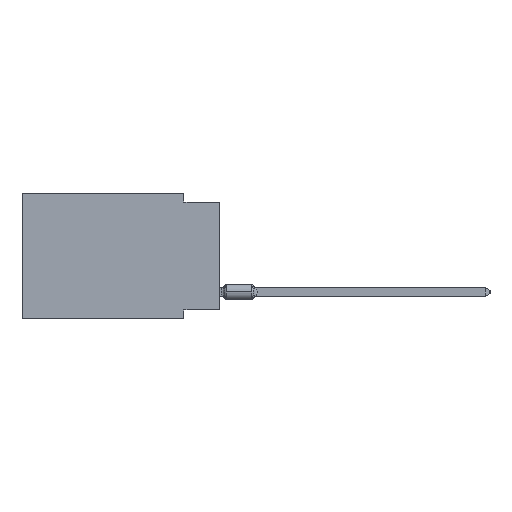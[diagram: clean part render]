
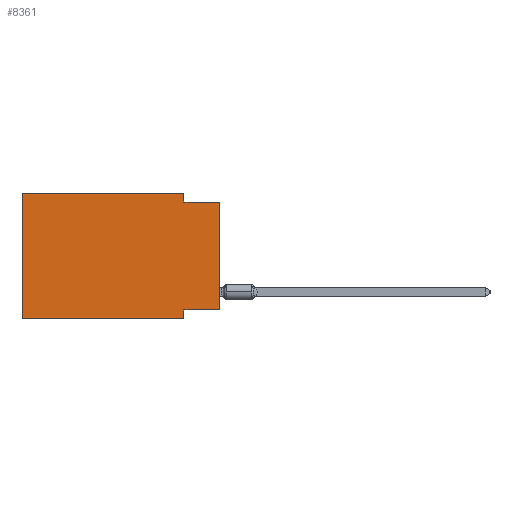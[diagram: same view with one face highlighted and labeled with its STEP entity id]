
A CAD part, left-side view. The second image highlights one B-rep face of the part: STEP entity #8361.
In plain terms, the highlighted planar face has unit normal (-1, 0, 0).
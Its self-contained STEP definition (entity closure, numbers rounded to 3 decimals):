
#645 = CARTESIAN_POINT ( 'NONE',  ( 0., 13.97, 0. ) ) ;
#853 = VERTEX_POINT ( 'NONE', #16847 ) ;
#8361 = ADVANCED_FACE ( 'NONE', ( #31615 ), #17648, .F. ) ;
#8714 = ORIENTED_EDGE ( 'NONE', *, *, #82675, .F. ) ;
#8896 = LINE ( 'NONE', #38214, #15114 ) ;
#10444 = DIRECTION ( 'NONE',  ( 0., -1., 0. ) ) ;
#12498 = VERTEX_POINT ( 'NONE', #42478 ) ;
#15114 = VECTOR ( 'NONE', #44915, 1000. ) ;
#16812 = CARTESIAN_POINT ( 'NONE',  ( 0., 2.54, -0.635 ) ) ;
#16847 = CARTESIAN_POINT ( 'NONE',  ( 0., 2.54, -8.89 ) ) ;
#17648 = PLANE ( 'NONE',  #80894 ) ;
#18167 = LINE ( 'NONE', #92196, #26492 ) ;
#18285 = CARTESIAN_POINT ( 'NONE',  ( 0., 2.54, -8.89 ) ) ;
#18522 = VECTOR ( 'NONE', #79520, 1000. ) ;
#21194 = DIRECTION ( 'NONE',  ( 0., 0., 1. ) ) ;
#21712 = ORIENTED_EDGE ( 'NONE', *, *, #71536, .F. ) ;
#26492 = VECTOR ( 'NONE', #47941, 1000. ) ;
#26695 = VECTOR ( 'NONE', #54966, 1000. ) ;
#28000 = CARTESIAN_POINT ( 'NONE',  ( 0., 0., -0.635 ) ) ;
#29479 = CARTESIAN_POINT ( 'NONE',  ( 0., 13.97, -8.89 ) ) ;
#30672 = CARTESIAN_POINT ( 'NONE',  ( 0., 13.97, -8.89 ) ) ;
#31040 = EDGE_CURVE ( 'NONE', #41817, #72069, #8896, .T. ) ;
#31063 = VERTEX_POINT ( 'NONE', #31460 ) ;
#31460 = CARTESIAN_POINT ( 'NONE',  ( 0., 2.54, 0. ) ) ;
#31615 = FACE_OUTER_BOUND ( 'NONE', #59789, .T. ) ;
#32337 = VECTOR ( 'NONE', #63117, 1000. ) ;
#34935 = CARTESIAN_POINT ( 'NONE',  ( 0., 13.97, 0. ) ) ;
#35223 = LINE ( 'NONE', #28000, #32337 ) ;
#38214 = CARTESIAN_POINT ( 'NONE',  ( 0., 13.97, 0. ) ) ;
#41817 = VERTEX_POINT ( 'NONE', #30672 ) ;
#42478 = CARTESIAN_POINT ( 'NONE',  ( 0., 2.54, -8.255 ) ) ;
#44915 = DIRECTION ( 'NONE',  ( 0., 0., 1. ) ) ;
#45713 = ORIENTED_EDGE ( 'NONE', *, *, #48249, .F. ) ;
#47765 = ORIENTED_EDGE ( 'NONE', *, *, #78366, .T. ) ;
#47941 = DIRECTION ( 'NONE',  ( 0., 1., 0. ) ) ;
#48249 = EDGE_CURVE ( 'NONE', #72069, #31063, #83504, .T. ) ;
#48394 = DIRECTION ( 'NONE',  ( 1., 0., 0. ) ) ;
#48626 = EDGE_CURVE ( 'NONE', #92317, #70538, #35223, .T. ) ;
#49755 = ORIENTED_EDGE ( 'NONE', *, *, #31040, .F. ) ;
#49796 = DIRECTION ( 'NONE',  ( 0., 0., -1. ) ) ;
#51533 = VERTEX_POINT ( 'NONE', #65725 ) ;
#52655 = VECTOR ( 'NONE', #75048, 1000. ) ;
#53529 = CARTESIAN_POINT ( 'NONE',  ( 0., 2.54, 0. ) ) ;
#53701 = CARTESIAN_POINT ( 'NONE',  ( 0., 13.97, 0. ) ) ;
#54966 = DIRECTION ( 'NONE',  ( 0., 0., -1. ) ) ;
#58596 = EDGE_CURVE ( 'NONE', #51533, #70538, #73563, .T. ) ;
#59789 = EDGE_LOOP ( 'NONE', ( #88439, #79707, #88510, #45713, #49755, #47765, #8714, #21712 ) ) ;
#61432 = VECTOR ( 'NONE', #10444, 1000. ) ;
#61665 = CARTESIAN_POINT ( 'NONE',  ( 0., 0., -0.635 ) ) ;
#63117 = DIRECTION ( 'NONE',  ( 0., -1., 0. ) ) ;
#64993 = VECTOR ( 'NONE', #21194, 1000. ) ;
#65725 = CARTESIAN_POINT ( 'NONE',  ( 0., 0., -8.255 ) ) ;
#68782 = LINE ( 'NONE', #18285, #52655 ) ;
#70538 = VERTEX_POINT ( 'NONE', #61665 ) ;
#71536 = EDGE_CURVE ( 'NONE', #51533, #12498, #18167, .T. ) ;
#72069 = VERTEX_POINT ( 'NONE', #645 ) ;
#73563 = LINE ( 'NONE', #87060, #64993 ) ;
#74659 = EDGE_CURVE ( 'NONE', #31063, #92317, #75170, .T. ) ;
#75048 = DIRECTION ( 'NONE',  ( 0., 0., -1. ) ) ;
#75170 = LINE ( 'NONE', #53529, #26695 ) ;
#78366 = EDGE_CURVE ( 'NONE', #41817, #853, #86726, .T. ) ;
#79520 = DIRECTION ( 'NONE',  ( 0., -1., 0. ) ) ;
#79707 = ORIENTED_EDGE ( 'NONE', *, *, #48626, .F. ) ;
#80894 = AXIS2_PLACEMENT_3D ( 'NONE', #34935, #48394, #49796 ) ;
#82675 = EDGE_CURVE ( 'NONE', #12498, #853, #68782, .T. ) ;
#83504 = LINE ( 'NONE', #53701, #61432 ) ;
#86726 = LINE ( 'NONE', #29479, #18522 ) ;
#87060 = CARTESIAN_POINT ( 'NONE',  ( 0., 0., 0. ) ) ;
#88439 = ORIENTED_EDGE ( 'NONE', *, *, #58596, .T. ) ;
#88510 = ORIENTED_EDGE ( 'NONE', *, *, #74659, .F. ) ;
#92196 = CARTESIAN_POINT ( 'NONE',  ( 0., 0., -8.255 ) ) ;
#92317 = VERTEX_POINT ( 'NONE', #16812 ) ;
